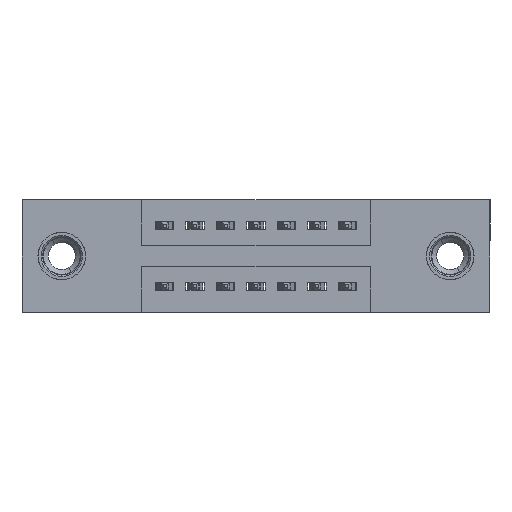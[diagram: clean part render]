
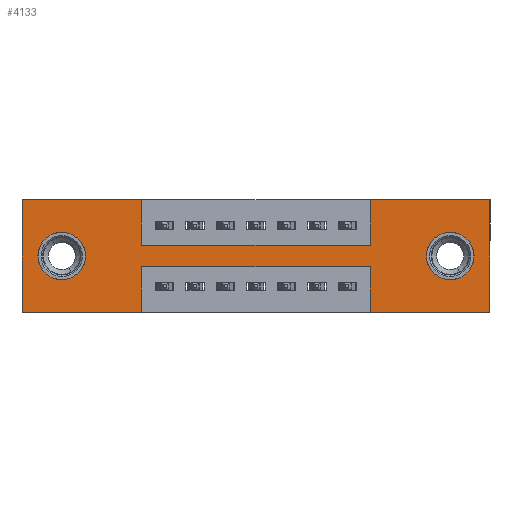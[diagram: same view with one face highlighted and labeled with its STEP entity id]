
A CAD part, front view. The second image highlights one B-rep face of the part: STEP entity #4133.
In plain terms, the highlighted planar face has unit normal (0, -1, 0).
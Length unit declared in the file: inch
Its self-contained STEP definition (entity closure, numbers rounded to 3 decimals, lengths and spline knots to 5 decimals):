
#349 = EDGE_CURVE ( 'NONE', #3731, #4515, #8010, .T. ) ;
#602 = CIRCLE ( 'NONE', #4352, 0.078 ) ;
#650 = EDGE_CURVE ( 'NONE', #901, #7862, #13835, .T. ) ;
#901 = VERTEX_POINT ( 'NONE', #8334 ) ;
#912 = VERTEX_POINT ( 'NONE', #7216 ) ;
#1151 = AXIS2_PLACEMENT_3D ( 'NONE', #6667, #5492, #6718 ) ;
#1176 = CARTESIAN_POINT ( 'NONE',  ( 0.13, 0., -0.185 ) ) ;
#1217 = EDGE_CURVE ( 'NONE', #6485, #13712, #602, .T. ) ;
#1292 = DIRECTION ( 'NONE',  ( 1., 0., 0. ) ) ;
#1328 = DIRECTION ( 'NONE',  ( 0., 0., 1. ) ) ;
#1489 = VECTOR ( 'NONE', #9447, 39.37008 ) ;
#1623 = CARTESIAN_POINT ( 'NONE',  ( 0., 0., -0.37 ) ) ;
#1686 = CARTESIAN_POINT ( 'NONE',  ( 0., 0., 0. ) ) ;
#2136 = VECTOR ( 'NONE', #8422, 39.37008 ) ;
#2279 = VECTOR ( 'NONE', #11082, 39.37008 ) ;
#2701 = ORIENTED_EDGE ( 'NONE', *, *, #12834, .T. ) ;
#2713 = EDGE_CURVE ( 'NONE', #13208, #11398, #6547, .T. ) ;
#2731 = PLANE ( 'NONE',  #8004 ) ;
#2841 = LINE ( 'NONE', #10641, #10100 ) ;
#2896 = DIRECTION ( 'NONE',  ( 0., 1., 0. ) ) ;
#2964 = CARTESIAN_POINT ( 'NONE',  ( 0.3925, 0., -0.15 ) ) ;
#2993 = CARTESIAN_POINT ( 'NONE',  ( 0., 0., -0.37 ) ) ;
#3063 = LINE ( 'NONE', #3502, #10492 ) ;
#3079 = CARTESIAN_POINT ( 'NONE',  ( 1.535, 0., -0.37 ) ) ;
#3093 = DIRECTION ( 'NONE',  ( 1., 0., 0. ) ) ;
#3305 = CARTESIAN_POINT ( 'NONE',  ( 0.13, 0., -0.107 ) ) ;
#3337 = EDGE_CURVE ( 'NONE', #3862, #912, #7430, .T. ) ;
#3484 = VECTOR ( 'NONE', #4198, 39.37008 ) ;
#3502 = CARTESIAN_POINT ( 'NONE',  ( 1.535, 0., 0. ) ) ;
#3579 = ORIENTED_EDGE ( 'NONE', *, *, #14007, .F. ) ;
#3731 = VERTEX_POINT ( 'NONE', #10022 ) ;
#3811 = ORIENTED_EDGE ( 'NONE', *, *, #349, .F. ) ;
#3862 = VERTEX_POINT ( 'NONE', #4851 ) ;
#4133 = ADVANCED_FACE ( 'NONE', ( #4867, #13782, #7591 ), #2731, .T. ) ;
#4198 = DIRECTION ( 'NONE',  ( 0., 0., 1. ) ) ;
#4325 = CARTESIAN_POINT ( 'NONE',  ( 0.3925, 0., -0.15 ) ) ;
#4352 = AXIS2_PLACEMENT_3D ( 'NONE', #1176, #13831, #9303 ) ;
#4501 = CARTESIAN_POINT ( 'NONE',  ( 1.405, 0., -0.185 ) ) ;
#4515 = VERTEX_POINT ( 'NONE', #6903 ) ;
#4851 = CARTESIAN_POINT ( 'NONE',  ( 0., 0., -0.37 ) ) ;
#4867 = FACE_BOUND ( 'NONE', #14808, .T. ) ;
#4969 = EDGE_CURVE ( 'NONE', #9601, #13488, #2841, .T. ) ;
#4972 = VECTOR ( 'NONE', #6484, 39.37008 ) ;
#5054 = DIRECTION ( 'NONE',  ( 0., 0., -1. ) ) ;
#5156 = ORIENTED_EDGE ( 'NONE', *, *, #9325, .F. ) ;
#5205 = LINE ( 'NONE', #1623, #2136 ) ;
#5256 = VECTOR ( 'NONE', #14244, 39.37008 ) ;
#5492 = DIRECTION ( 'NONE',  ( 0., 1., 0. ) ) ;
#5718 = EDGE_CURVE ( 'NONE', #912, #7961, #14062, .T. ) ;
#5832 = EDGE_CURVE ( 'NONE', #4515, #3862, #8587, .T. ) ;
#5841 = CARTESIAN_POINT ( 'NONE',  ( 0.3925, 0., -0.22 ) ) ;
#5978 = LINE ( 'NONE', #8820, #12347 ) ;
#6126 = ORIENTED_EDGE ( 'NONE', *, *, #5718, .F. ) ;
#6171 = VECTOR ( 'NONE', #3093, 39.37008 ) ;
#6413 = LINE ( 'NONE', #5841, #1489 ) ;
#6484 = DIRECTION ( 'NONE',  ( -1., 0., 0. ) ) ;
#6485 = VERTEX_POINT ( 'NONE', #6542 ) ;
#6542 = CARTESIAN_POINT ( 'NONE',  ( 0.13, 0., -0.263 ) ) ;
#6547 = CIRCLE ( 'NONE', #11526, 0.078 ) ;
#6654 = ORIENTED_EDGE ( 'NONE', *, *, #3337, .F. ) ;
#6667 = CARTESIAN_POINT ( 'NONE',  ( 0.13, 0., -0.185 ) ) ;
#6718 = DIRECTION ( 'NONE',  ( 0., 0., 1. ) ) ;
#6727 = CARTESIAN_POINT ( 'NONE',  ( 0.3925, 0., 0. ) ) ;
#6745 = LINE ( 'NONE', #4325, #6171 ) ;
#6903 = CARTESIAN_POINT ( 'NONE',  ( 0.3925, 0., -0.37 ) ) ;
#7216 = CARTESIAN_POINT ( 'NONE',  ( 0., 0., 0. ) ) ;
#7430 = LINE ( 'NONE', #1686, #5256 ) ;
#7591 = FACE_OUTER_BOUND ( 'NONE', #10070, .T. ) ;
#7623 = ORIENTED_EDGE ( 'NONE', *, *, #8711, .F. ) ;
#7634 = VERTEX_POINT ( 'NONE', #2964 ) ;
#7646 = ORIENTED_EDGE ( 'NONE', *, *, #5832, .F. ) ;
#7802 = CARTESIAN_POINT ( 'NONE',  ( 1.1425, 0., 0. ) ) ;
#7862 = VERTEX_POINT ( 'NONE', #7802 ) ;
#7961 = VERTEX_POINT ( 'NONE', #6727 ) ;
#8004 = AXIS2_PLACEMENT_3D ( 'NONE', #2993, #13285, #12274 ) ;
#8007 = EDGE_CURVE ( 'NONE', #7961, #7634, #5978, .T. ) ;
#8010 = LINE ( 'NONE', #14218, #12780 ) ;
#8279 = ORIENTED_EDGE ( 'NONE', *, *, #650, .F. ) ;
#8334 = CARTESIAN_POINT ( 'NONE',  ( 1.1425, 0., -0.15 ) ) ;
#8422 = DIRECTION ( 'NONE',  ( -1., 0., 0. ) ) ;
#8587 = LINE ( 'NONE', #14579, #4972 ) ;
#8711 = EDGE_CURVE ( 'NONE', #10086, #8877, #3063, .T. ) ;
#8738 = CARTESIAN_POINT ( 'NONE',  ( 1.405, 0., -0.263 ) ) ;
#8820 = CARTESIAN_POINT ( 'NONE',  ( 0.3925, 0., 0. ) ) ;
#8877 = VERTEX_POINT ( 'NONE', #3079 ) ;
#9197 = ORIENTED_EDGE ( 'NONE', *, *, #2713, .T. ) ;
#9303 = DIRECTION ( 'NONE',  ( 0., 0., 1. ) ) ;
#9325 = EDGE_CURVE ( 'NONE', #8877, #9601, #5205, .T. ) ;
#9444 = ORIENTED_EDGE ( 'NONE', *, *, #13741, .T. ) ;
#9447 = DIRECTION ( 'NONE',  ( -1., 0., 0. ) ) ;
#9453 = CARTESIAN_POINT ( 'NONE',  ( 0., 0., 0. ) ) ;
#9542 = VECTOR ( 'NONE', #1292, 39.37008 ) ;
#9601 = VERTEX_POINT ( 'NONE', #14456 ) ;
#9724 = EDGE_LOOP ( 'NONE', ( #9444, #12860 ) ) ;
#9930 = LINE ( 'NONE', #9453, #9542 ) ;
#9988 = DIRECTION ( 'NONE',  ( 0., 0., -1. ) ) ;
#10022 = CARTESIAN_POINT ( 'NONE',  ( 0.3925, 0., -0.22 ) ) ;
#10070 = EDGE_LOOP ( 'NONE', ( #3811, #11523, #13212, #5156, #7623, #13770, #8279, #3579, #12388, #6126, #6654, #7646 ) ) ;
#10086 = VERTEX_POINT ( 'NONE', #11223 ) ;
#10100 = VECTOR ( 'NONE', #1328, 39.37008 ) ;
#10407 = CARTESIAN_POINT ( 'NONE',  ( 1.405, 0., -0.107 ) ) ;
#10492 = VECTOR ( 'NONE', #10987, 39.37008 ) ;
#10641 = CARTESIAN_POINT ( 'NONE',  ( 1.1425, 0., -0.37 ) ) ;
#10987 = DIRECTION ( 'NONE',  ( 0., 0., -1. ) ) ;
#11082 = DIRECTION ( 'NONE',  ( 1., 0., 0. ) ) ;
#11153 = DIRECTION ( 'NONE',  ( 0., 0., -1. ) ) ;
#11223 = CARTESIAN_POINT ( 'NONE',  ( 1.535, 0., 0. ) ) ;
#11398 = VERTEX_POINT ( 'NONE', #8738 ) ;
#11523 = ORIENTED_EDGE ( 'NONE', *, *, #12693, .F. ) ;
#11526 = AXIS2_PLACEMENT_3D ( 'NONE', #4501, #13773, #11584 ) ;
#11584 = DIRECTION ( 'NONE',  ( 0., 0., -1. ) ) ;
#12036 = CARTESIAN_POINT ( 'NONE',  ( 0., 0., 0. ) ) ;
#12123 = CARTESIAN_POINT ( 'NONE',  ( 1.405, 0., -0.185 ) ) ;
#12255 = CARTESIAN_POINT ( 'NONE',  ( 1.1425, 0., 0. ) ) ;
#12274 = DIRECTION ( 'NONE',  ( 0., 0., -1. ) ) ;
#12347 = VECTOR ( 'NONE', #9988, 39.37008 ) ;
#12388 = ORIENTED_EDGE ( 'NONE', *, *, #8007, .F. ) ;
#12693 = EDGE_CURVE ( 'NONE', #13488, #3731, #6413, .T. ) ;
#12780 = VECTOR ( 'NONE', #5054, 39.37008 ) ;
#12834 = EDGE_CURVE ( 'NONE', #11398, #13208, #14176, .T. ) ;
#12860 = ORIENTED_EDGE ( 'NONE', *, *, #1217, .T. ) ;
#13208 = VERTEX_POINT ( 'NONE', #10407 ) ;
#13212 = ORIENTED_EDGE ( 'NONE', *, *, #4969, .F. ) ;
#13285 = DIRECTION ( 'NONE',  ( 0., -1., 0. ) ) ;
#13488 = VERTEX_POINT ( 'NONE', #14547 ) ;
#13637 = CIRCLE ( 'NONE', #1151, 0.078 ) ;
#13662 = AXIS2_PLACEMENT_3D ( 'NONE', #12123, #2896, #11153 ) ;
#13712 = VERTEX_POINT ( 'NONE', #3305 ) ;
#13741 = EDGE_CURVE ( 'NONE', #13712, #6485, #13637, .T. ) ;
#13770 = ORIENTED_EDGE ( 'NONE', *, *, #14903, .F. ) ;
#13773 = DIRECTION ( 'NONE',  ( 0., 1., 0. ) ) ;
#13782 = FACE_BOUND ( 'NONE', #9724, .T. ) ;
#13831 = DIRECTION ( 'NONE',  ( 0., 1., 0. ) ) ;
#13835 = LINE ( 'NONE', #12255, #3484 ) ;
#14007 = EDGE_CURVE ( 'NONE', #7634, #901, #6745, .T. ) ;
#14062 = LINE ( 'NONE', #12036, #2279 ) ;
#14176 = CIRCLE ( 'NONE', #13662, 0.078 ) ;
#14218 = CARTESIAN_POINT ( 'NONE',  ( 0.3925, 0., -0.37 ) ) ;
#14244 = DIRECTION ( 'NONE',  ( 0., 0., 1. ) ) ;
#14456 = CARTESIAN_POINT ( 'NONE',  ( 1.1425, 0., -0.37 ) ) ;
#14547 = CARTESIAN_POINT ( 'NONE',  ( 1.1425, 0., -0.22 ) ) ;
#14579 = CARTESIAN_POINT ( 'NONE',  ( 0., 0., -0.37 ) ) ;
#14808 = EDGE_LOOP ( 'NONE', ( #9197, #2701 ) ) ;
#14903 = EDGE_CURVE ( 'NONE', #7862, #10086, #9930, .T. ) ;
